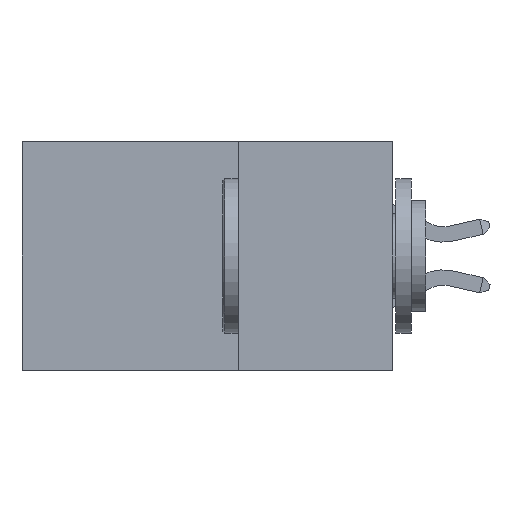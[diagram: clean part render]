
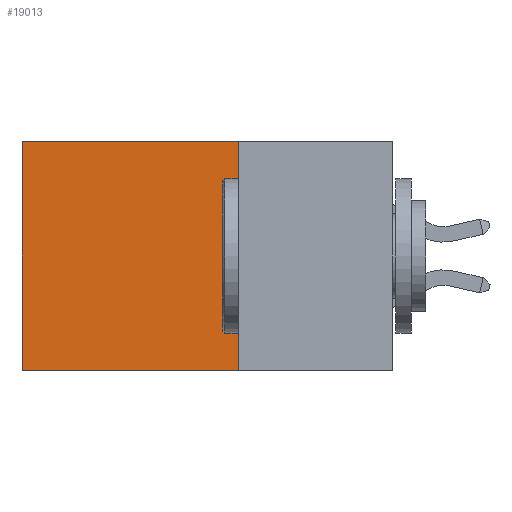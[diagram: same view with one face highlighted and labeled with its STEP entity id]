
A CAD part, left-side view. The second image highlights one B-rep face of the part: STEP entity #19013.
In plain terms, the highlighted planar face has unit normal (-1, 0, 0).
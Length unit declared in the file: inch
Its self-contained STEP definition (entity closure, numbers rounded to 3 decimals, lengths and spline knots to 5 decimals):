
#562 = CARTESIAN_POINT ( 'NONE',  ( 0.2875, 0.25, -0.37 ) ) ;
#683 = CARTESIAN_POINT ( 'NONE',  ( 0.2875, 0.25, 0. ) ) ;
#1185 = EDGE_CURVE ( 'NONE', #6108, #14989, #17275, .T. ) ;
#1847 = CARTESIAN_POINT ( 'NONE',  ( 0.2875, 0.25, 0. ) ) ;
#2996 = DIRECTION ( 'NONE',  ( 0., 1., 0. ) ) ;
#3355 = CARTESIAN_POINT ( 'NONE',  ( 0.2875, 0.25, 0. ) ) ;
#3621 = CARTESIAN_POINT ( 'NONE',  ( 0.2875, 0.25, 0. ) ) ;
#3812 = ORIENTED_EDGE ( 'NONE', *, *, #23305, .T. ) ;
#5205 = VERTEX_POINT ( 'NONE', #3621 ) ;
#6108 = VERTEX_POINT ( 'NONE', #562 ) ;
#6133 = FACE_OUTER_BOUND ( 'NONE', #24228, .T. ) ;
#10665 = EDGE_CURVE ( 'NONE', #5205, #20023, #22481, .T. ) ;
#10710 = VECTOR ( 'NONE', #12442, 39.37008 ) ;
#10855 = PLANE ( 'NONE',  #15008 ) ;
#11668 = CARTESIAN_POINT ( 'NONE',  ( 0.2875, 0.6, 0. ) ) ;
#12442 = DIRECTION ( 'NONE',  ( 0., 0., -1. ) ) ;
#12644 = EDGE_CURVE ( 'NONE', #5205, #6108, #14652, .T. ) ;
#12674 = LINE ( 'NONE', #11668, #13377 ) ;
#13377 = VECTOR ( 'NONE', #27442, 39.37008 ) ;
#14652 = LINE ( 'NONE', #3355, #10710 ) ;
#14989 = VERTEX_POINT ( 'NONE', #21588 ) ;
#15008 = AXIS2_PLACEMENT_3D ( 'NONE', #1847, #26920, #22033 ) ;
#15172 = ORIENTED_EDGE ( 'NONE', *, *, #10665, .T. ) ;
#17275 = LINE ( 'NONE', #28880, #18724 ) ;
#18532 = CARTESIAN_POINT ( 'NONE',  ( 0.2875, 0.6, 0. ) ) ;
#18724 = VECTOR ( 'NONE', #19933, 39.37008 ) ;
#19013 = ADVANCED_FACE ( 'NONE', ( #6133 ), #10855, .F. ) ;
#19933 = DIRECTION ( 'NONE',  ( 0., 1., 0. ) ) ;
#20023 = VERTEX_POINT ( 'NONE', #18532 ) ;
#21588 = CARTESIAN_POINT ( 'NONE',  ( 0.2875, 0.6, -0.37 ) ) ;
#22033 = DIRECTION ( 'NONE',  ( 0., 0., -1. ) ) ;
#22481 = LINE ( 'NONE', #683, #26332 ) ;
#23060 = ORIENTED_EDGE ( 'NONE', *, *, #12644, .F. ) ;
#23305 = EDGE_CURVE ( 'NONE', #20023, #14989, #12674, .T. ) ;
#24228 = EDGE_LOOP ( 'NONE', ( #3812, #24796, #23060, #15172 ) ) ;
#24796 = ORIENTED_EDGE ( 'NONE', *, *, #1185, .F. ) ;
#26332 = VECTOR ( 'NONE', #2996, 39.37008 ) ;
#26920 = DIRECTION ( 'NONE',  ( 1., 0., 0. ) ) ;
#27442 = DIRECTION ( 'NONE',  ( 0., 0., -1. ) ) ;
#28880 = CARTESIAN_POINT ( 'NONE',  ( 0.2875, 0.25, -0.37 ) ) ;
